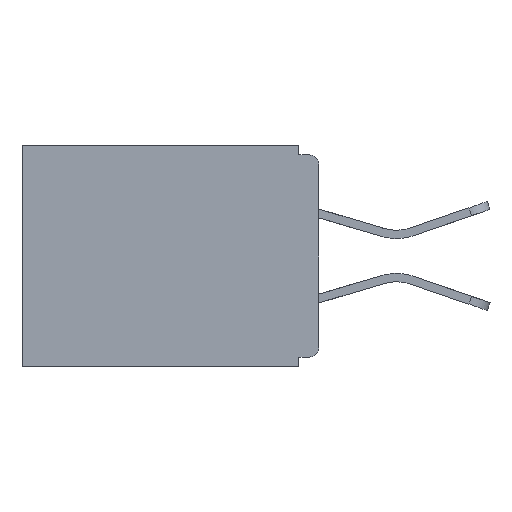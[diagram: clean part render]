
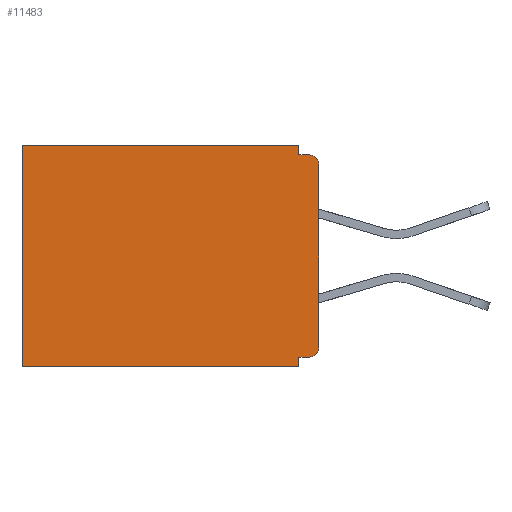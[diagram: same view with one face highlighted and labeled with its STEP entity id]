
A CAD part, left-side view. The second image highlights one B-rep face of the part: STEP entity #11483.
In plain terms, the highlighted planar face has unit normal (-1, 0, 0).
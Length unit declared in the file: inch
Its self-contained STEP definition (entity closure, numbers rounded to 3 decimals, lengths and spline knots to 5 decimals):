
#221 = ORIENTED_EDGE ( 'NONE', *, *, #3018, .T. ) ;
#455 = VERTEX_POINT ( 'NONE', #19559 ) ;
#586 = CARTESIAN_POINT ( 'NONE',  ( 0.298, 0.015, -0.313 ) ) ;
#716 = FACE_OUTER_BOUND ( 'NONE', #5982, .T. ) ;
#857 = DIRECTION ( 'NONE',  ( 0., 1., 0. ) ) ;
#1001 = ORIENTED_EDGE ( 'NONE', *, *, #11622, .F. ) ;
#1363 = CARTESIAN_POINT ( 'NONE',  ( 0.298, 0., -0.015 ) ) ;
#1403 = AXIS2_PLACEMENT_3D ( 'NONE', #586, #7596, #18821 ) ;
#1465 = CIRCLE ( 'NONE', #15394, 0.015 ) ;
#1584 = CARTESIAN_POINT ( 'NONE',  ( 0.298, 0., 0. ) ) ;
#1786 = LINE ( 'NONE', #14992, #17995 ) ;
#2406 = CARTESIAN_POINT ( 'NONE',  ( 0.298, 0.015, -0.03 ) ) ;
#2991 = VERTEX_POINT ( 'NONE', #13779 ) ;
#3018 = EDGE_CURVE ( 'NONE', #455, #20464, #18506, .T. ) ;
#4354 = EDGE_CURVE ( 'NONE', #20464, #20717, #10811, .T. ) ;
#5028 = PLANE ( 'NONE',  #19961 ) ;
#5370 = VECTOR ( 'NONE', #8770, 39.37008 ) ;
#5841 = LINE ( 'NONE', #1363, #8586 ) ;
#5982 = EDGE_LOOP ( 'NONE', ( #18305, #9244, #17569, #221, #16496, #8268, #1001, #7464, #11278, #18627 ) ) ;
#6603 = EDGE_CURVE ( 'NONE', #15680, #20717, #20577, .T. ) ;
#6904 = CARTESIAN_POINT ( 'NONE',  ( 0.298, 0.031, -0.328 ) ) ;
#7132 = DIRECTION ( 'NONE',  ( 0., 0., -1. ) ) ;
#7418 = CARTESIAN_POINT ( 'NONE',  ( 0.298, 0.46, -0.343 ) ) ;
#7464 = ORIENTED_EDGE ( 'NONE', *, *, #20495, .F. ) ;
#7596 = DIRECTION ( 'NONE',  ( -1., 0., 0. ) ) ;
#8268 = ORIENTED_EDGE ( 'NONE', *, *, #6603, .F. ) ;
#8586 = VECTOR ( 'NONE', #13629, 39.37008 ) ;
#8664 = DIRECTION ( 'NONE',  ( 0., 1., 0. ) ) ;
#8766 = VERTEX_POINT ( 'NONE', #18884 ) ;
#8770 = DIRECTION ( 'NONE',  ( 0., 1., 0. ) ) ;
#9244 = ORIENTED_EDGE ( 'NONE', *, *, #13822, .F. ) ;
#9634 = CARTESIAN_POINT ( 'NONE',  ( 0.298, 0., -0.343 ) ) ;
#10344 = CARTESIAN_POINT ( 'NONE',  ( 0.298, 0.031, -0.343 ) ) ;
#10811 = LINE ( 'NONE', #22370, #19306 ) ;
#11277 = DIRECTION ( 'NONE',  ( 0., 0., -1. ) ) ;
#11278 = ORIENTED_EDGE ( 'NONE', *, *, #11328, .T. ) ;
#11328 = EDGE_CURVE ( 'NONE', #19531, #2991, #21889, .T. ) ;
#11483 = ADVANCED_FACE ( 'NONE', ( #716 ), #5028, .F. ) ;
#11622 = EDGE_CURVE ( 'NONE', #11996, #15680, #14977, .T. ) ;
#11848 = DIRECTION ( 'NONE',  ( 0., 0., -1. ) ) ;
#11996 = VERTEX_POINT ( 'NONE', #6904 ) ;
#12313 = DIRECTION ( 'NONE',  ( 0., 0., -1. ) ) ;
#12459 = VERTEX_POINT ( 'NONE', #16905 ) ;
#13629 = DIRECTION ( 'NONE',  ( 0., -1., 0. ) ) ;
#13779 = CARTESIAN_POINT ( 'NONE',  ( 0.298, 0., -0.313 ) ) ;
#13822 = EDGE_CURVE ( 'NONE', #12459, #20827, #5841, .T. ) ;
#13830 = CARTESIAN_POINT ( 'NONE',  ( 0.298, 0.46, 0. ) ) ;
#14731 = LINE ( 'NONE', #18681, #18546 ) ;
#14977 = LINE ( 'NONE', #16880, #15842 ) ;
#14992 = CARTESIAN_POINT ( 'NONE',  ( 0.298, 0., 0. ) ) ;
#15068 = DIRECTION ( 'NONE',  ( 0., 0., -1. ) ) ;
#15394 = AXIS2_PLACEMENT_3D ( 'NONE', #2406, #16604, #11277 ) ;
#15680 = VERTEX_POINT ( 'NONE', #16622 ) ;
#15697 = DIRECTION ( 'NONE',  ( 1., 0., 0. ) ) ;
#15842 = VECTOR ( 'NONE', #16738, 39.37008 ) ;
#16151 = CARTESIAN_POINT ( 'NONE',  ( 0.298, 0.015, -0.015 ) ) ;
#16496 = ORIENTED_EDGE ( 'NONE', *, *, #4354, .T. ) ;
#16604 = DIRECTION ( 'NONE',  ( -1., 0., 0. ) ) ;
#16622 = CARTESIAN_POINT ( 'NONE',  ( 0.298, 0.031, -0.343 ) ) ;
#16738 = DIRECTION ( 'NONE',  ( 0., 0., -1. ) ) ;
#16880 = CARTESIAN_POINT ( 'NONE',  ( 0.298, 0.031, -0.343 ) ) ;
#16905 = CARTESIAN_POINT ( 'NONE',  ( 0.298, 0.031, -0.015 ) ) ;
#17276 = CARTESIAN_POINT ( 'NONE',  ( 0.298, 0., 0. ) ) ;
#17448 = LINE ( 'NONE', #10344, #20472 ) ;
#17569 = ORIENTED_EDGE ( 'NONE', *, *, #17779, .F. ) ;
#17779 = EDGE_CURVE ( 'NONE', #455, #12459, #17448, .T. ) ;
#17995 = VECTOR ( 'NONE', #15068, 39.37008 ) ;
#18213 = EDGE_CURVE ( 'NONE', #8766, #2991, #1786, .T. ) ;
#18305 = ORIENTED_EDGE ( 'NONE', *, *, #18907, .T. ) ;
#18506 = LINE ( 'NONE', #1584, #5370 ) ;
#18546 = VECTOR ( 'NONE', #8664, 39.37008 ) ;
#18627 = ORIENTED_EDGE ( 'NONE', *, *, #18213, .F. ) ;
#18681 = CARTESIAN_POINT ( 'NONE',  ( 0.298, 0., -0.328 ) ) ;
#18821 = DIRECTION ( 'NONE',  ( 0., 0., -1. ) ) ;
#18884 = CARTESIAN_POINT ( 'NONE',  ( 0.298, 0., -0.03 ) ) ;
#18907 = EDGE_CURVE ( 'NONE', #8766, #20827, #1465, .T. ) ;
#18913 = VECTOR ( 'NONE', #857, 39.37008 ) ;
#19306 = VECTOR ( 'NONE', #11848, 39.37008 ) ;
#19531 = VERTEX_POINT ( 'NONE', #22731 ) ;
#19559 = CARTESIAN_POINT ( 'NONE',  ( 0.298, 0.031, 0. ) ) ;
#19961 = AXIS2_PLACEMENT_3D ( 'NONE', #17276, #15697, #7132 ) ;
#20464 = VERTEX_POINT ( 'NONE', #13830 ) ;
#20472 = VECTOR ( 'NONE', #12313, 39.37008 ) ;
#20495 = EDGE_CURVE ( 'NONE', #19531, #11996, #14731, .T. ) ;
#20577 = LINE ( 'NONE', #9634, #18913 ) ;
#20717 = VERTEX_POINT ( 'NONE', #7418 ) ;
#20827 = VERTEX_POINT ( 'NONE', #16151 ) ;
#21889 = CIRCLE ( 'NONE', #1403, 0.015 ) ;
#22370 = CARTESIAN_POINT ( 'NONE',  ( 0.298, 0.46, 0. ) ) ;
#22731 = CARTESIAN_POINT ( 'NONE',  ( 0.298, 0.015, -0.328 ) ) ;
